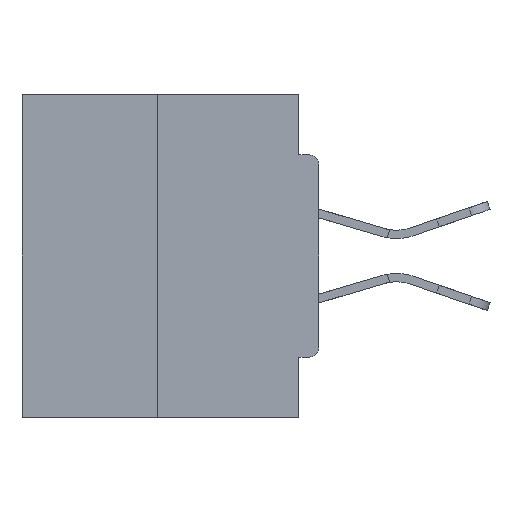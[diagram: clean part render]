
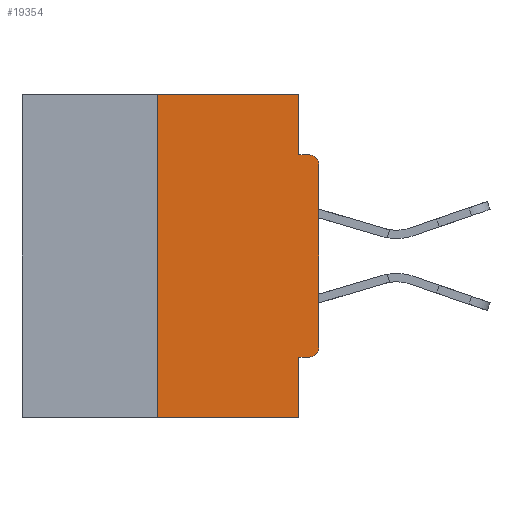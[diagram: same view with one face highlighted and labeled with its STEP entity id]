
A CAD part, left-side view. The second image highlights one B-rep face of the part: STEP entity #19354.
In plain terms, the highlighted planar face has unit normal (-1, 0, 0).
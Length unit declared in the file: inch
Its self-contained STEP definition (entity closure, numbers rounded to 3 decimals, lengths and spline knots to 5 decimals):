
#24 = ORIENTED_EDGE ( 'NONE', *, *, #5634, .F. ) ;
#689 = CARTESIAN_POINT ( 'NONE',  ( 0., 0., -0.4065 ) ) ;
#1287 = DIRECTION ( 'NONE',  ( 0., 0., -1. ) ) ;
#1738 = CIRCLE ( 'NONE', #7128, 0.015 ) ;
#1961 = DIRECTION ( 'NONE',  ( 0., -1., 0. ) ) ;
#2183 = CARTESIAN_POINT ( 'NONE',  ( 0., 0.25, 0. ) ) ;
#2279 = ORIENTED_EDGE ( 'NONE', *, *, #18044, .F. ) ;
#2283 = CARTESIAN_POINT ( 'NONE',  ( 0., 0.031, -0.5 ) ) ;
#2445 = DIRECTION ( 'NONE',  ( 0., 0., -1. ) ) ;
#3470 = CARTESIAN_POINT ( 'NONE',  ( 0., 0.46, 0. ) ) ;
#3863 = DIRECTION ( 'NONE',  ( -1., 0., 0. ) ) ;
#4146 = CARTESIAN_POINT ( 'NONE',  ( 0., 0.031, 0. ) ) ;
#4568 = CARTESIAN_POINT ( 'NONE',  ( 0., 0.031, -0.5 ) ) ;
#5634 = EDGE_CURVE ( 'NONE', #34521, #30936, #17383, .T. ) ;
#5957 = EDGE_CURVE ( 'NONE', #26696, #29723, #13069, .T. ) ;
#6056 = LINE ( 'NONE', #16012, #8104 ) ;
#6589 = LINE ( 'NONE', #8335, #28775 ) ;
#6738 = ORIENTED_EDGE ( 'NONE', *, *, #5957, .T. ) ;
#7128 = AXIS2_PLACEMENT_3D ( 'NONE', #24537, #8857, #16827 ) ;
#7362 = VECTOR ( 'NONE', #8908, 39.37008 ) ;
#7392 = CARTESIAN_POINT ( 'NONE',  ( 0., 0., -0.1085 ) ) ;
#7472 = LINE ( 'NONE', #28507, #16727 ) ;
#7644 = ORIENTED_EDGE ( 'NONE', *, *, #10009, .F. ) ;
#8104 = VECTOR ( 'NONE', #29445, 39.37008 ) ;
#8335 = CARTESIAN_POINT ( 'NONE',  ( 0., 0.46, -0.5 ) ) ;
#8857 = DIRECTION ( 'NONE',  ( -1., 0., 0. ) ) ;
#8908 = DIRECTION ( 'NONE',  ( 0., 0., -1. ) ) ;
#9051 = ORIENTED_EDGE ( 'NONE', *, *, #10057, .F. ) ;
#9068 = DIRECTION ( 'NONE',  ( 0., 0., -1. ) ) ;
#9491 = VERTEX_POINT ( 'NONE', #33617 ) ;
#9746 = EDGE_CURVE ( 'NONE', #10607, #30936, #6589, .T. ) ;
#10009 = EDGE_CURVE ( 'NONE', #19445, #17766, #30450, .T. ) ;
#10057 = EDGE_CURVE ( 'NONE', #17766, #29723, #14968, .T. ) ;
#10207 = AXIS2_PLACEMENT_3D ( 'NONE', #3470, #25163, #1287 ) ;
#10227 = VECTOR ( 'NONE', #2445, 39.37008 ) ;
#10607 = VERTEX_POINT ( 'NONE', #23689 ) ;
#12095 = LINE ( 'NONE', #20003, #28844 ) ;
#13069 = CIRCLE ( 'NONE', #21760, 0.015 ) ;
#13189 = ORIENTED_EDGE ( 'NONE', *, *, #9746, .T. ) ;
#13257 = VECTOR ( 'NONE', #1961, 39.37008 ) ;
#13553 = EDGE_LOOP ( 'NONE', ( #2279, #33273, #13189, #24, #23215, #25668, #19016, #6738, #9051, #7644 ) ) ;
#14062 = PLANE ( 'NONE',  #10207 ) ;
#14757 = CARTESIAN_POINT ( 'NONE',  ( 0., 0.031, 0. ) ) ;
#14968 = LINE ( 'NONE', #17580, #13257 ) ;
#15465 = EDGE_CURVE ( 'NONE', #24665, #26696, #6056, .T. ) ;
#16012 = CARTESIAN_POINT ( 'NONE',  ( 0., 0., 0. ) ) ;
#16727 = VECTOR ( 'NONE', #20239, 39.37008 ) ;
#16827 = DIRECTION ( 'NONE',  ( 0., 0., -1. ) ) ;
#17383 = LINE ( 'NONE', #2283, #10227 ) ;
#17580 = CARTESIAN_POINT ( 'NONE',  ( 0., 0., -0.0935 ) ) ;
#17766 = VERTEX_POINT ( 'NONE', #24073 ) ;
#18031 = CARTESIAN_POINT ( 'NONE',  ( 0., 0.031, -0.4065 ) ) ;
#18044 = EDGE_CURVE ( 'NONE', #23576, #19445, #12095, .T. ) ;
#18155 = EDGE_CURVE ( 'NONE', #10607, #23576, #7472, .T. ) ;
#18559 = LINE ( 'NONE', #689, #33615 ) ;
#19016 = ORIENTED_EDGE ( 'NONE', *, *, #15465, .T. ) ;
#19354 = ADVANCED_FACE ( 'NONE', ( #23282 ), #14062, .F. ) ;
#19445 = VERTEX_POINT ( 'NONE', #4146 ) ;
#20003 = CARTESIAN_POINT ( 'NONE',  ( 0., 0.46, 0. ) ) ;
#20239 = DIRECTION ( 'NONE',  ( 0., 0., 1. ) ) ;
#21760 = AXIS2_PLACEMENT_3D ( 'NONE', #28133, #3863, #9068 ) ;
#22080 = DIRECTION ( 'NONE',  ( 0., -1., 0. ) ) ;
#22707 = EDGE_CURVE ( 'NONE', #9491, #24665, #1738, .T. ) ;
#23215 = ORIENTED_EDGE ( 'NONE', *, *, #29752, .F. ) ;
#23282 = FACE_OUTER_BOUND ( 'NONE', #13553, .T. ) ;
#23576 = VERTEX_POINT ( 'NONE', #2183 ) ;
#23689 = CARTESIAN_POINT ( 'NONE',  ( 0., 0.25, -0.5 ) ) ;
#24073 = CARTESIAN_POINT ( 'NONE',  ( 0., 0.031, -0.0935 ) ) ;
#24537 = CARTESIAN_POINT ( 'NONE',  ( 0., 0.015, -0.3915 ) ) ;
#24665 = VERTEX_POINT ( 'NONE', #34177 ) ;
#25163 = DIRECTION ( 'NONE',  ( 1., 0., 0. ) ) ;
#25668 = ORIENTED_EDGE ( 'NONE', *, *, #22707, .T. ) ;
#26696 = VERTEX_POINT ( 'NONE', #7392 ) ;
#26888 = CARTESIAN_POINT ( 'NONE',  ( 0., 0.015, -0.0935 ) ) ;
#28133 = CARTESIAN_POINT ( 'NONE',  ( 0., 0.015, -0.1085 ) ) ;
#28507 = CARTESIAN_POINT ( 'NONE',  ( 0., 0.25, 0. ) ) ;
#28775 = VECTOR ( 'NONE', #22080, 39.37008 ) ;
#28844 = VECTOR ( 'NONE', #30408, 39.37008 ) ;
#29445 = DIRECTION ( 'NONE',  ( 0., 0., 1. ) ) ;
#29723 = VERTEX_POINT ( 'NONE', #26888 ) ;
#29752 = EDGE_CURVE ( 'NONE', #9491, #34521, #18559, .T. ) ;
#30408 = DIRECTION ( 'NONE',  ( 0., -1., 0. ) ) ;
#30450 = LINE ( 'NONE', #14757, #7362 ) ;
#30936 = VERTEX_POINT ( 'NONE', #4568 ) ;
#32628 = DIRECTION ( 'NONE',  ( 0., 1., 0. ) ) ;
#33273 = ORIENTED_EDGE ( 'NONE', *, *, #18155, .F. ) ;
#33615 = VECTOR ( 'NONE', #32628, 39.37008 ) ;
#33617 = CARTESIAN_POINT ( 'NONE',  ( 0., 0.015, -0.4065 ) ) ;
#34177 = CARTESIAN_POINT ( 'NONE',  ( 0., 0., -0.3915 ) ) ;
#34521 = VERTEX_POINT ( 'NONE', #18031 ) ;
